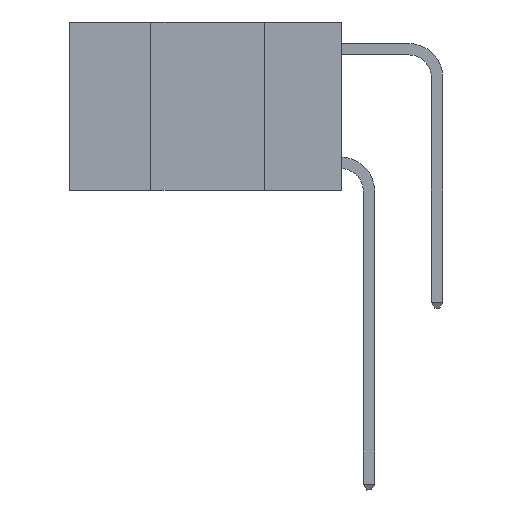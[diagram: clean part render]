
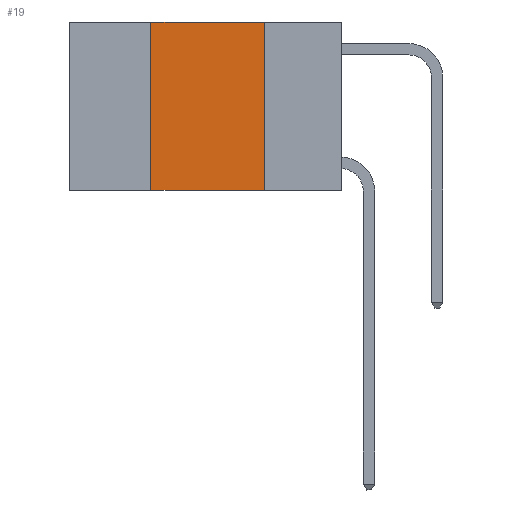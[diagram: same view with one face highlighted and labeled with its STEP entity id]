
A CAD part, left-side view. The second image highlights one B-rep face of the part: STEP entity #19.
In plain terms, the highlighted planar face has unit normal (-1, 0, 0).
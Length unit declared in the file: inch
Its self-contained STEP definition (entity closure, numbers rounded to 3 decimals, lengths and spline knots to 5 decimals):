
#19 = ADVANCED_FACE ( 'NONE', ( #9473 ), #2108, .F. ) ;
#205 = CARTESIAN_POINT ( 'NONE',  ( 0., 0.42, 0. ) ) ;
#439 = DIRECTION ( 'NONE',  ( 0., -1., 0. ) ) ;
#852 = EDGE_CURVE ( 'NONE', #7882, #9923, #5435, .T. ) ;
#860 = ORIENTED_EDGE ( 'NONE', *, *, #4684, .F. ) ;
#904 = VECTOR ( 'NONE', #439, 39.37008 ) ;
#1026 = EDGE_LOOP ( 'NONE', ( #860, #5670, #9218, #4187 ) ) ;
#1503 = CARTESIAN_POINT ( 'NONE',  ( 0., 0.6, -0.37 ) ) ;
#1606 = LINE ( 'NONE', #8678, #3929 ) ;
#1697 = VERTEX_POINT ( 'NONE', #6439 ) ;
#2108 = PLANE ( 'NONE',  #9004 ) ;
#2237 = CARTESIAN_POINT ( 'NONE',  ( 0., 0.42, -0.37 ) ) ;
#2724 = CARTESIAN_POINT ( 'NONE',  ( 0., 0.6, 0. ) ) ;
#2800 = EDGE_CURVE ( 'NONE', #7882, #6785, #8980, .T. ) ;
#3929 = VECTOR ( 'NONE', #7677, 39.37008 ) ;
#4041 = LINE ( 'NONE', #2724, #904 ) ;
#4187 = ORIENTED_EDGE ( 'NONE', *, *, #852, .T. ) ;
#4518 = DIRECTION ( 'NONE',  ( 0., 0., -1. ) ) ;
#4549 = VECTOR ( 'NONE', #5380, 39.37008 ) ;
#4684 = EDGE_CURVE ( 'NONE', #1697, #9923, #1606, .T. ) ;
#4886 = CARTESIAN_POINT ( 'NONE',  ( 0., 0.17, -0.37 ) ) ;
#5300 = CARTESIAN_POINT ( 'NONE',  ( 0., 0.6, 0. ) ) ;
#5380 = DIRECTION ( 'NONE',  ( 0., -1., 0. ) ) ;
#5420 = EDGE_CURVE ( 'NONE', #6785, #1697, #4041, .T. ) ;
#5435 = LINE ( 'NONE', #1503, #4549 ) ;
#5670 = ORIENTED_EDGE ( 'NONE', *, *, #5420, .F. ) ;
#6439 = CARTESIAN_POINT ( 'NONE',  ( 0., 0.17, 0. ) ) ;
#6714 = CARTESIAN_POINT ( 'NONE',  ( 0., 0.42, 0. ) ) ;
#6785 = VERTEX_POINT ( 'NONE', #205 ) ;
#7677 = DIRECTION ( 'NONE',  ( 0., 0., -1. ) ) ;
#7882 = VERTEX_POINT ( 'NONE', #2237 ) ;
#8466 = DIRECTION ( 'NONE',  ( 1., 0., 0. ) ) ;
#8678 = CARTESIAN_POINT ( 'NONE',  ( 0., 0.17, 0. ) ) ;
#8980 = LINE ( 'NONE', #6714, #10188 ) ;
#9004 = AXIS2_PLACEMENT_3D ( 'NONE', #5300, #8466, #4518 ) ;
#9175 = DIRECTION ( 'NONE',  ( 0., 0., 1. ) ) ;
#9218 = ORIENTED_EDGE ( 'NONE', *, *, #2800, .F. ) ;
#9473 = FACE_OUTER_BOUND ( 'NONE', #1026, .T. ) ;
#9923 = VERTEX_POINT ( 'NONE', #4886 ) ;
#10188 = VECTOR ( 'NONE', #9175, 39.37008 ) ;
